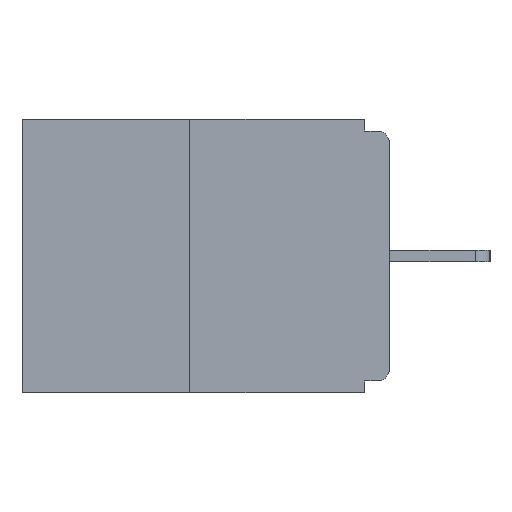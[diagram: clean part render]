
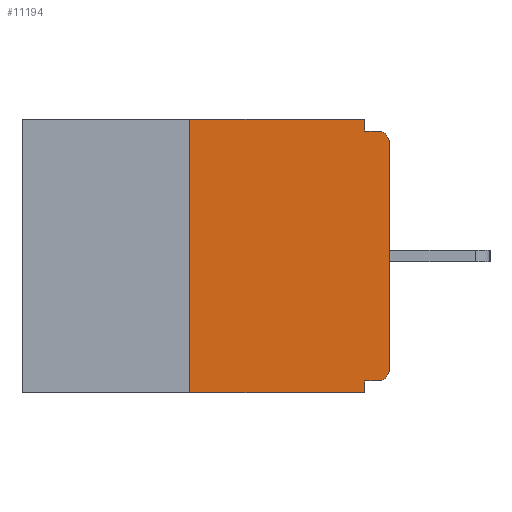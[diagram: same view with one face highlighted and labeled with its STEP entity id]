
A CAD part, left-side view. The second image highlights one B-rep face of the part: STEP entity #11194.
In plain terms, the highlighted planar face has unit normal (-1, 0, 0).
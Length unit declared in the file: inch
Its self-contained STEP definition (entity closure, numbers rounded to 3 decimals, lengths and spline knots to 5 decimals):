
#199 = CARTESIAN_POINT ( 'NONE',  ( 0., 0.46, -0.343 ) ) ;
#207 = EDGE_CURVE ( 'NONE', #2725, #12632, #1172, .T. ) ;
#458 = ORIENTED_EDGE ( 'NONE', *, *, #13313, .F. ) ;
#479 = DIRECTION ( 'NONE',  ( 0., 0., -1. ) ) ;
#923 = CARTESIAN_POINT ( 'NONE',  ( 0., 0., -0.015 ) ) ;
#1172 = LINE ( 'NONE', #10340, #8572 ) ;
#1261 = AXIS2_PLACEMENT_3D ( 'NONE', #5846, #6791, #479 ) ;
#1310 = EDGE_CURVE ( 'NONE', #3186, #7509, #11220, .T. ) ;
#1333 = VECTOR ( 'NONE', #14701, 39.37008 ) ;
#1715 = CARTESIAN_POINT ( 'NONE',  ( 0., 0.015, -0.328 ) ) ;
#2343 = FACE_OUTER_BOUND ( 'NONE', #5959, .T. ) ;
#2370 = CIRCLE ( 'NONE', #1261, 0.015 ) ;
#2418 = CARTESIAN_POINT ( 'NONE',  ( 0., 0.031, -0.015 ) ) ;
#2435 = CARTESIAN_POINT ( 'NONE',  ( 0., 0., -0.313 ) ) ;
#2503 = CARTESIAN_POINT ( 'NONE',  ( 0., 0.46, 0. ) ) ;
#2573 = ORIENTED_EDGE ( 'NONE', *, *, #1310, .F. ) ;
#2725 = VERTEX_POINT ( 'NONE', #2435 ) ;
#3043 = EDGE_CURVE ( 'NONE', #14204, #10116, #8661, .T. ) ;
#3159 = CARTESIAN_POINT ( 'NONE',  ( 0., 0.031, 0. ) ) ;
#3186 = VERTEX_POINT ( 'NONE', #2418 ) ;
#3900 = VERTEX_POINT ( 'NONE', #11550 ) ;
#4311 = DIRECTION ( 'NONE',  ( 0., 0., -1. ) ) ;
#4627 = ORIENTED_EDGE ( 'NONE', *, *, #7649, .T. ) ;
#4637 = DIRECTION ( 'NONE',  ( 0., -1., 0. ) ) ;
#5003 = EDGE_CURVE ( 'NONE', #14204, #2725, #15281, .T. ) ;
#5186 = DIRECTION ( 'NONE',  ( 0., 0., -1. ) ) ;
#5224 = EDGE_CURVE ( 'NONE', #7738, #3900, #9358, .T. ) ;
#5618 = LINE ( 'NONE', #10903, #1333 ) ;
#5846 = CARTESIAN_POINT ( 'NONE',  ( 0., 0.015, -0.03 ) ) ;
#5959 = EDGE_LOOP ( 'NONE', ( #12059, #14592, #16590, #10576, #14673, #15317, #11064, #4627, #2573, #458 ) ) ;
#5975 = VECTOR ( 'NONE', #4637, 39.37008 ) ;
#6180 = VECTOR ( 'NONE', #4311, 39.37008 ) ;
#6769 = DIRECTION ( 'NONE',  ( 0., -1., 0. ) ) ;
#6791 = DIRECTION ( 'NONE',  ( -1., 0., 0. ) ) ;
#7451 = VERTEX_POINT ( 'NONE', #8619 ) ;
#7453 = CARTESIAN_POINT ( 'NONE',  ( 0., 0.46, 0. ) ) ;
#7509 = VERTEX_POINT ( 'NONE', #16990 ) ;
#7576 = DIRECTION ( 'NONE',  ( 0., 0., -1. ) ) ;
#7649 = EDGE_CURVE ( 'NONE', #12632, #7509, #2370, .T. ) ;
#7738 = VERTEX_POINT ( 'NONE', #8427 ) ;
#8427 = CARTESIAN_POINT ( 'NONE',  ( 0., 0.25, -0.343 ) ) ;
#8572 = VECTOR ( 'NONE', #11814, 39.37008 ) ;
#8619 = CARTESIAN_POINT ( 'NONE',  ( 0., 0.25, 0. ) ) ;
#8661 = LINE ( 'NONE', #12737, #15547 ) ;
#9358 = LINE ( 'NONE', #199, #10303 ) ;
#10055 = CARTESIAN_POINT ( 'NONE',  ( 0., 0.031, -0.343 ) ) ;
#10116 = VERTEX_POINT ( 'NONE', #12089 ) ;
#10303 = VECTOR ( 'NONE', #6769, 39.37008 ) ;
#10340 = CARTESIAN_POINT ( 'NONE',  ( 0., 0., 0. ) ) ;
#10399 = DIRECTION ( 'NONE',  ( 0., -1., 0. ) ) ;
#10576 = ORIENTED_EDGE ( 'NONE', *, *, #13965, .F. ) ;
#10635 = VERTEX_POINT ( 'NONE', #3159 ) ;
#10724 = CARTESIAN_POINT ( 'NONE',  ( 0., 0., -0.03 ) ) ;
#10764 = EDGE_CURVE ( 'NONE', #7451, #10635, #17036, .T. ) ;
#10903 = CARTESIAN_POINT ( 'NONE',  ( 0., 0.25, 0. ) ) ;
#11064 = ORIENTED_EDGE ( 'NONE', *, *, #207, .T. ) ;
#11194 = ADVANCED_FACE ( 'NONE', ( #2343 ), #11442, .F. ) ;
#11220 = LINE ( 'NONE', #923, #5975 ) ;
#11405 = DIRECTION ( 'NONE',  ( -1., 0., 0. ) ) ;
#11442 = PLANE ( 'NONE',  #12766 ) ;
#11550 = CARTESIAN_POINT ( 'NONE',  ( 0., 0.031, -0.343 ) ) ;
#11814 = DIRECTION ( 'NONE',  ( 0., 0., 1. ) ) ;
#12059 = ORIENTED_EDGE ( 'NONE', *, *, #10764, .F. ) ;
#12089 = CARTESIAN_POINT ( 'NONE',  ( 0., 0.031, -0.328 ) ) ;
#12182 = CARTESIAN_POINT ( 'NONE',  ( 0., 0.031, 0. ) ) ;
#12632 = VERTEX_POINT ( 'NONE', #10724 ) ;
#12737 = CARTESIAN_POINT ( 'NONE',  ( 0., 0., -0.328 ) ) ;
#12766 = AXIS2_PLACEMENT_3D ( 'NONE', #2503, #14116, #12829 ) ;
#12829 = DIRECTION ( 'NONE',  ( 0., 0., -1. ) ) ;
#13223 = VECTOR ( 'NONE', #5186, 39.37008 ) ;
#13313 = EDGE_CURVE ( 'NONE', #10635, #3186, #15202, .T. ) ;
#13957 = DIRECTION ( 'NONE',  ( 0., 1., 0. ) ) ;
#13965 = EDGE_CURVE ( 'NONE', #10116, #3900, #16431, .T. ) ;
#14116 = DIRECTION ( 'NONE',  ( 1., 0., 0. ) ) ;
#14151 = EDGE_CURVE ( 'NONE', #7738, #7451, #5618, .T. ) ;
#14176 = CARTESIAN_POINT ( 'NONE',  ( 0., 0.015, -0.313 ) ) ;
#14204 = VERTEX_POINT ( 'NONE', #1715 ) ;
#14592 = ORIENTED_EDGE ( 'NONE', *, *, #14151, .F. ) ;
#14673 = ORIENTED_EDGE ( 'NONE', *, *, #3043, .F. ) ;
#14701 = DIRECTION ( 'NONE',  ( 0., 0., 1. ) ) ;
#15202 = LINE ( 'NONE', #12182, #6180 ) ;
#15281 = CIRCLE ( 'NONE', #16896, 0.015 ) ;
#15317 = ORIENTED_EDGE ( 'NONE', *, *, #5003, .T. ) ;
#15547 = VECTOR ( 'NONE', #13957, 39.37008 ) ;
#15762 = VECTOR ( 'NONE', #10399, 39.37008 ) ;
#16431 = LINE ( 'NONE', #10055, #13223 ) ;
#16590 = ORIENTED_EDGE ( 'NONE', *, *, #5224, .T. ) ;
#16896 = AXIS2_PLACEMENT_3D ( 'NONE', #14176, #11405, #7576 ) ;
#16990 = CARTESIAN_POINT ( 'NONE',  ( 0., 0.015, -0.015 ) ) ;
#17036 = LINE ( 'NONE', #7453, #15762 ) ;
